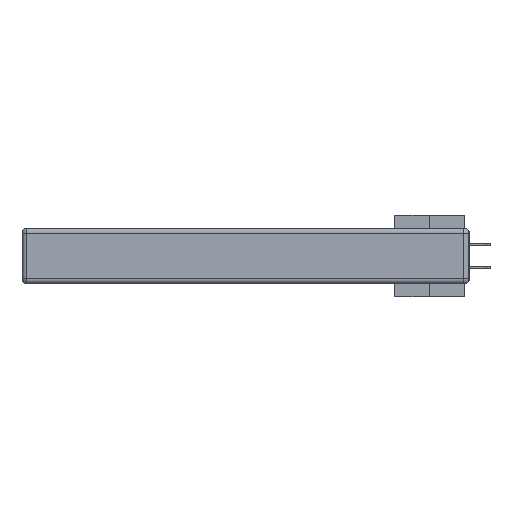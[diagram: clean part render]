
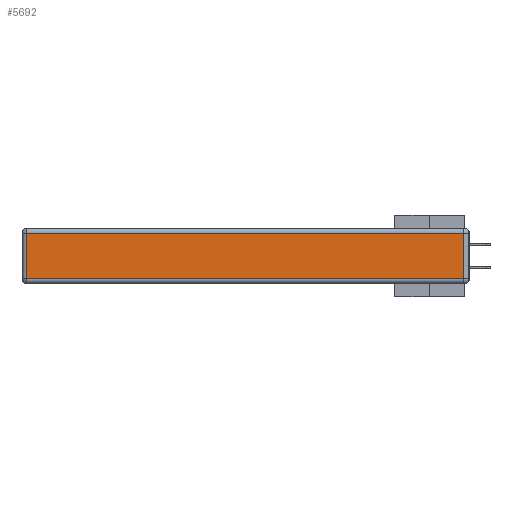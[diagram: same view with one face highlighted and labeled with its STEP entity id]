
A CAD part, left-side view. The second image highlights one B-rep face of the part: STEP entity #5692.
In plain terms, the highlighted planar face has unit normal (-1, 0, 0).
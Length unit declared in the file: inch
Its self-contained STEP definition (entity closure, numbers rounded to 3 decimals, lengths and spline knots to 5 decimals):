
#3024 = CARTESIAN_POINT ( 'NONE',  ( 0., 0., -0.313 ) ) ;
#5270 = CARTESIAN_POINT ( 'NONE',  ( 0., 0.03, -0.313 ) ) ;
#5692 = ADVANCED_FACE ( 'NONE', ( #16866 ), #28450, .T. ) ;
#7096 = EDGE_LOOP ( 'NONE', ( #7222, #15045, #41203, #22250 ) ) ;
#7222 = ORIENTED_EDGE ( 'NONE', *, *, #8727, .T. ) ;
#8468 = AXIS2_PLACEMENT_3D ( 'NONE', #24823, #35310, #38536 ) ;
#8727 = EDGE_CURVE ( 'NONE', #25506, #12141, #18648, .T. ) ;
#8829 = VECTOR ( 'NONE', #37035, 39.37008 ) ;
#9783 = VECTOR ( 'NONE', #33380, 39.37008 ) ;
#10221 = EDGE_CURVE ( 'NONE', #20668, #25506, #27217, .T. ) ;
#12029 = CARTESIAN_POINT ( 'NONE',  ( 0., 2.72, -0.03 ) ) ;
#12141 = VERTEX_POINT ( 'NONE', #5270 ) ;
#14286 = CARTESIAN_POINT ( 'NONE',  ( 0., 2.72, -0.313 ) ) ;
#14451 = VECTOR ( 'NONE', #22945, 39.37008 ) ;
#15045 = ORIENTED_EDGE ( 'NONE', *, *, #40720, .T. ) ;
#16866 = FACE_OUTER_BOUND ( 'NONE', #7096, .T. ) ;
#17102 = CARTESIAN_POINT ( 'NONE',  ( 0., 2.75, -0.03 ) ) ;
#18648 = LINE ( 'NONE', #3024, #9783 ) ;
#20668 = VERTEX_POINT ( 'NONE', #12029 ) ;
#22250 = ORIENTED_EDGE ( 'NONE', *, *, #10221, .T. ) ;
#22945 = DIRECTION ( 'NONE',  ( 0., 0., 1. ) ) ;
#24823 = CARTESIAN_POINT ( 'NONE',  ( 0., 0., -0.343 ) ) ;
#25506 = VERTEX_POINT ( 'NONE', #14286 ) ;
#25622 = VERTEX_POINT ( 'NONE', #42823 ) ;
#26488 = DIRECTION ( 'NONE',  ( 0., 0., -1. ) ) ;
#27217 = LINE ( 'NONE', #30185, #36070 ) ;
#28450 = PLANE ( 'NONE',  #8468 ) ;
#29174 = EDGE_CURVE ( 'NONE', #25622, #20668, #31833, .T. ) ;
#30185 = CARTESIAN_POINT ( 'NONE',  ( 0., 2.72, -0.343 ) ) ;
#31833 = LINE ( 'NONE', #17102, #8829 ) ;
#32903 = CARTESIAN_POINT ( 'NONE',  ( 0., 0.03, -0.343 ) ) ;
#33380 = DIRECTION ( 'NONE',  ( 0., -1., 0. ) ) ;
#35310 = DIRECTION ( 'NONE',  ( -1., 0., 0. ) ) ;
#36070 = VECTOR ( 'NONE', #26488, 39.37008 ) ;
#37035 = DIRECTION ( 'NONE',  ( 0., 1., 0. ) ) ;
#37383 = LINE ( 'NONE', #32903, #14451 ) ;
#38536 = DIRECTION ( 'NONE',  ( 0., 0., 1. ) ) ;
#40720 = EDGE_CURVE ( 'NONE', #12141, #25622, #37383, .T. ) ;
#41203 = ORIENTED_EDGE ( 'NONE', *, *, #29174, .T. ) ;
#42823 = CARTESIAN_POINT ( 'NONE',  ( 0., 0.03, -0.03 ) ) ;
